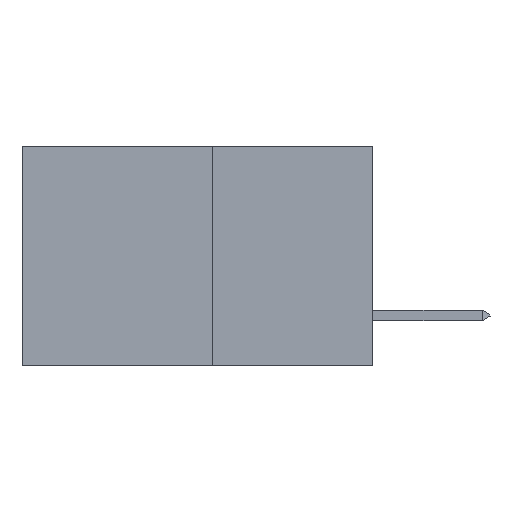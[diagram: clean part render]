
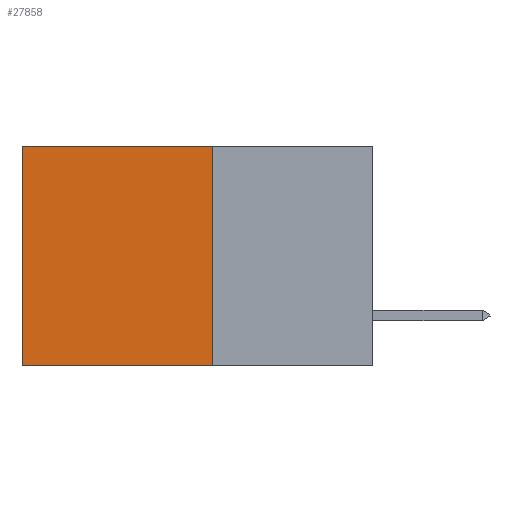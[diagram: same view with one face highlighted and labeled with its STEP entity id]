
A CAD part, left-side view. The second image highlights one B-rep face of the part: STEP entity #27858.
In plain terms, the highlighted planar face has unit normal (-1, 0, 0).
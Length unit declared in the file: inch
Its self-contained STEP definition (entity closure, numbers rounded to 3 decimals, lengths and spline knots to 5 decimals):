
#1644 = CARTESIAN_POINT ( 'NONE',  ( 0.277, 0.59, 0. ) ) ;
#1894 = PLANE ( 'NONE',  #16920 ) ;
#3087 = VECTOR ( 'NONE', #12491, 39.37008 ) ;
#4595 = VERTEX_POINT ( 'NONE', #24093 ) ;
#5978 = LINE ( 'NONE', #32147, #12104 ) ;
#7266 = CARTESIAN_POINT ( 'NONE',  ( 0.277, 0.27, -0.37 ) ) ;
#9410 = CARTESIAN_POINT ( 'NONE',  ( 0.277, 0.27, -0.37 ) ) ;
#9888 = DIRECTION ( 'NONE',  ( 0., 0., -1. ) ) ;
#11132 = VERTEX_POINT ( 'NONE', #31095 ) ;
#11866 = EDGE_CURVE ( 'NONE', #4595, #32205, #17007, .T. ) ;
#12104 = VECTOR ( 'NONE', #21656, 39.37008 ) ;
#12491 = DIRECTION ( 'NONE',  ( 0., 1., 0. ) ) ;
#12901 = CARTESIAN_POINT ( 'NONE',  ( 0.277, 0.27, 0. ) ) ;
#13820 = VECTOR ( 'NONE', #16658, 39.37008 ) ;
#15095 = EDGE_CURVE ( 'NONE', #32205, #11132, #33882, .T. ) ;
#16284 = EDGE_LOOP ( 'NONE', ( #20380, #33675, #32906, #29809 ) ) ;
#16658 = DIRECTION ( 'NONE',  ( 0., 0., -1. ) ) ;
#16920 = AXIS2_PLACEMENT_3D ( 'NONE', #7266, #25457, #9888 ) ;
#17007 = LINE ( 'NONE', #12901, #3087 ) ;
#17448 = EDGE_CURVE ( 'NONE', #4595, #26304, #30766, .T. ) ;
#20172 = DIRECTION ( 'NONE',  ( 0., 0., -1. ) ) ;
#20380 = ORIENTED_EDGE ( 'NONE', *, *, #15095, .T. ) ;
#20683 = FACE_OUTER_BOUND ( 'NONE', #16284, .T. ) ;
#21656 = DIRECTION ( 'NONE',  ( 0., 1., 0. ) ) ;
#23765 = VECTOR ( 'NONE', #20172, 39.37008 ) ;
#24093 = CARTESIAN_POINT ( 'NONE',  ( 0.277, 0.27, 0. ) ) ;
#25457 = DIRECTION ( 'NONE',  ( 1., 0., 0. ) ) ;
#26304 = VERTEX_POINT ( 'NONE', #9410 ) ;
#27858 = ADVANCED_FACE ( 'NONE', ( #20683 ), #1894, .F. ) ;
#27914 = CARTESIAN_POINT ( 'NONE',  ( 0.277, 0.27, -0.37 ) ) ;
#28723 = EDGE_CURVE ( 'NONE', #26304, #11132, #5978, .T. ) ;
#29809 = ORIENTED_EDGE ( 'NONE', *, *, #11866, .T. ) ;
#30766 = LINE ( 'NONE', #27914, #23765 ) ;
#31095 = CARTESIAN_POINT ( 'NONE',  ( 0.277, 0.59, -0.37 ) ) ;
#32147 = CARTESIAN_POINT ( 'NONE',  ( 0.277, 0.27, -0.37 ) ) ;
#32205 = VERTEX_POINT ( 'NONE', #1644 ) ;
#32373 = CARTESIAN_POINT ( 'NONE',  ( 0.277, 0.59, -0.37 ) ) ;
#32906 = ORIENTED_EDGE ( 'NONE', *, *, #17448, .F. ) ;
#33675 = ORIENTED_EDGE ( 'NONE', *, *, #28723, .F. ) ;
#33882 = LINE ( 'NONE', #32373, #13820 ) ;
